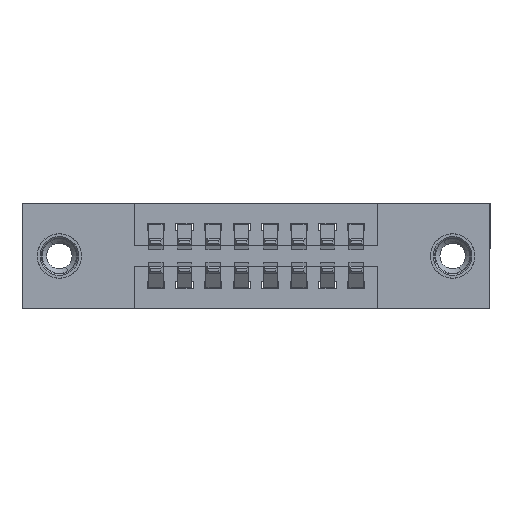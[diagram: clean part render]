
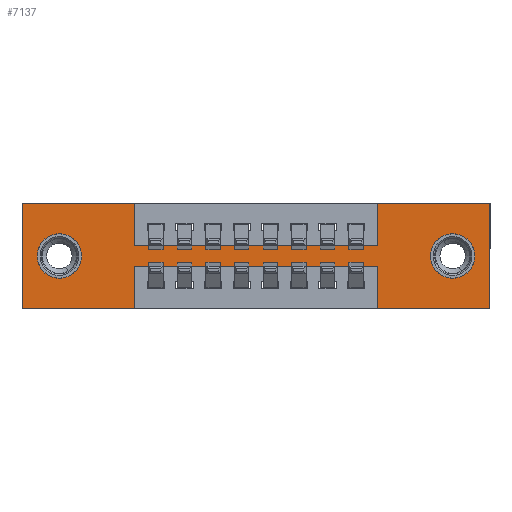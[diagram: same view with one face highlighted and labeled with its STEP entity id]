
A CAD part, front view. The second image highlights one B-rep face of the part: STEP entity #7137.
In plain terms, the highlighted planar face has unit normal (0, -1, 0).
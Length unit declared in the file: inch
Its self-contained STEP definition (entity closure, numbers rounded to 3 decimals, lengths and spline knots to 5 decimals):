
#36 = VECTOR ( 'NONE', #2842, 39.37008 ) ;
#48 = ORIENTED_EDGE ( 'NONE', *, *, #8321, .T. ) ;
#423 = CARTESIAN_POINT ( 'NONE',  ( 1.2425, 0., 0. ) ) ;
#436 = CARTESIAN_POINT ( 'NONE',  ( 0., 0., 0. ) ) ;
#591 = DIRECTION ( 'NONE',  ( 0., 0., 1. ) ) ;
#675 = VERTEX_POINT ( 'NONE', #4288 ) ;
#711 = CARTESIAN_POINT ( 'NONE',  ( 1.2425, 0., -0.22 ) ) ;
#812 = CARTESIAN_POINT ( 'NONE',  ( 0.3925, 0., -0.15 ) ) ;
#958 = CARTESIAN_POINT ( 'NONE',  ( 0.3925, 0., -0.37 ) ) ;
#1055 = EDGE_CURVE ( 'NONE', #2383, #12617, #11240, .T. ) ;
#1197 = VERTEX_POINT ( 'NONE', #436 ) ;
#1211 = DIRECTION ( 'NONE',  ( 0., 0., 1. ) ) ;
#1275 = CARTESIAN_POINT ( 'NONE',  ( 0.13, 0., -0.263 ) ) ;
#1289 = CARTESIAN_POINT ( 'NONE',  ( 0.3925, 0., -0.22 ) ) ;
#1409 = EDGE_CURVE ( 'NONE', #12295, #2345, #5709, .T. ) ;
#1460 = LINE ( 'NONE', #11836, #6264 ) ;
#1564 = DIRECTION ( 'NONE',  ( 1., 0., 0. ) ) ;
#1579 = ORIENTED_EDGE ( 'NONE', *, *, #4553, .F. ) ;
#1686 = ORIENTED_EDGE ( 'NONE', *, *, #5200, .F. ) ;
#1727 = DIRECTION ( 'NONE',  ( 0., 0., -1. ) ) ;
#1734 = FACE_BOUND ( 'NONE', #6515, .T. ) ;
#1882 = DIRECTION ( 'NONE',  ( 0., 0., -1. ) ) ;
#1994 = VECTOR ( 'NONE', #11374, 39.37008 ) ;
#1997 = CARTESIAN_POINT ( 'NONE',  ( 0., 0., -0.37 ) ) ;
#2053 = FACE_OUTER_BOUND ( 'NONE', #4636, .T. ) ;
#2105 = DIRECTION ( 'NONE',  ( -1., 0., 0. ) ) ;
#2143 = CARTESIAN_POINT ( 'NONE',  ( 1.2425, 0., 0. ) ) ;
#2266 = CARTESIAN_POINT ( 'NONE',  ( 0., 0., -0.37 ) ) ;
#2345 = VERTEX_POINT ( 'NONE', #8189 ) ;
#2347 = EDGE_CURVE ( 'NONE', #675, #11377, #6633, .T. ) ;
#2383 = VERTEX_POINT ( 'NONE', #6997 ) ;
#2524 = EDGE_CURVE ( 'NONE', #8164, #12295, #9024, .T. ) ;
#2536 = VECTOR ( 'NONE', #4565, 39.37008 ) ;
#2552 = DIRECTION ( 'NONE',  ( 0., 0., -1. ) ) ;
#2568 = CARTESIAN_POINT ( 'NONE',  ( 0., 0., 0. ) ) ;
#2617 = VECTOR ( 'NONE', #9044, 39.37008 ) ;
#2749 = DIRECTION ( 'NONE',  ( 0., 1., 0. ) ) ;
#2842 = DIRECTION ( 'NONE',  ( 0., 0., 1. ) ) ;
#2877 = AXIS2_PLACEMENT_3D ( 'NONE', #2935, #8913, #1882 ) ;
#2935 = CARTESIAN_POINT ( 'NONE',  ( 1.505, 0., -0.185 ) ) ;
#2956 = LINE ( 'NONE', #812, #2617 ) ;
#3151 = VERTEX_POINT ( 'NONE', #3806 ) ;
#3208 = VERTEX_POINT ( 'NONE', #2266 ) ;
#3241 = CIRCLE ( 'NONE', #2877, 0.078 ) ;
#3324 = CARTESIAN_POINT ( 'NONE',  ( 0.3925, 0., 0. ) ) ;
#3443 = ORIENTED_EDGE ( 'NONE', *, *, #10557, .T. ) ;
#3741 = EDGE_CURVE ( 'NONE', #6452, #8164, #2956, .T. ) ;
#3800 = DIRECTION ( 'NONE',  ( 1., 0., 0. ) ) ;
#3806 = CARTESIAN_POINT ( 'NONE',  ( 1.505, 0., -0.107 ) ) ;
#3946 = CIRCLE ( 'NONE', #6463, 0.078 ) ;
#4049 = EDGE_CURVE ( 'NONE', #2345, #675, #1460, .T. ) ;
#4132 = CARTESIAN_POINT ( 'NONE',  ( 0.3925, 0., -0.15 ) ) ;
#4146 = CARTESIAN_POINT ( 'NONE',  ( 0., 0., 0. ) ) ;
#4288 = CARTESIAN_POINT ( 'NONE',  ( 1.635, 0., -0.37 ) ) ;
#4373 = ORIENTED_EDGE ( 'NONE', *, *, #5862, .F. ) ;
#4392 = VERTEX_POINT ( 'NONE', #1275 ) ;
#4553 = EDGE_CURVE ( 'NONE', #11377, #7640, #10487, .T. ) ;
#4565 = DIRECTION ( 'NONE',  ( 0., 0., 1. ) ) ;
#4636 = EDGE_LOOP ( 'NONE', ( #6553, #10226, #1579, #6552, #11717, #11842, #8780, #10229, #5778, #13063, #4373, #1686 ) ) ;
#4665 = CARTESIAN_POINT ( 'NONE',  ( 0.3925, 0., 0. ) ) ;
#4873 = AXIS2_PLACEMENT_3D ( 'NONE', #7339, #5225, #11232 ) ;
#4968 = VERTEX_POINT ( 'NONE', #4665 ) ;
#4985 = CARTESIAN_POINT ( 'NONE',  ( 1.2425, 0., -0.15 ) ) ;
#5200 = EDGE_CURVE ( 'NONE', #12617, #3208, #5457, .T. ) ;
#5224 = CARTESIAN_POINT ( 'NONE',  ( 1.2425, 0., -0.37 ) ) ;
#5225 = DIRECTION ( 'NONE',  ( 0., -1., 0. ) ) ;
#5282 = CARTESIAN_POINT ( 'NONE',  ( 0., 0., -0.37 ) ) ;
#5457 = LINE ( 'NONE', #1997, #9731 ) ;
#5477 = CIRCLE ( 'NONE', #9786, 0.078 ) ;
#5508 = EDGE_CURVE ( 'NONE', #3151, #8769, #3241, .T. ) ;
#5697 = EDGE_LOOP ( 'NONE', ( #7759, #3443 ) ) ;
#5709 = LINE ( 'NONE', #2568, #8887 ) ;
#5765 = DIRECTION ( 'NONE',  ( 0., 1., 0. ) ) ;
#5778 = ORIENTED_EDGE ( 'NONE', *, *, #9629, .F. ) ;
#5862 = EDGE_CURVE ( 'NONE', #3208, #1197, #7328, .T. ) ;
#6264 = VECTOR ( 'NONE', #1727, 39.37008 ) ;
#6420 = CARTESIAN_POINT ( 'NONE',  ( 1.505, 0., -0.263 ) ) ;
#6452 = VERTEX_POINT ( 'NONE', #4132 ) ;
#6463 = AXIS2_PLACEMENT_3D ( 'NONE', #9794, #2749, #591 ) ;
#6515 = EDGE_LOOP ( 'NONE', ( #9899, #48 ) ) ;
#6552 = ORIENTED_EDGE ( 'NONE', *, *, #2347, .F. ) ;
#6553 = ORIENTED_EDGE ( 'NONE', *, *, #1055, .F. ) ;
#6633 = LINE ( 'NONE', #5282, #12322 ) ;
#6732 = CARTESIAN_POINT ( 'NONE',  ( 1.505, 0., -0.185 ) ) ;
#6997 = CARTESIAN_POINT ( 'NONE',  ( 0.3925, 0., -0.22 ) ) ;
#7137 = ADVANCED_FACE ( 'NONE', ( #1734, #9849, #2053 ), #7248, .T. ) ;
#7248 = PLANE ( 'NONE',  #4873 ) ;
#7328 = LINE ( 'NONE', #7796, #36 ) ;
#7335 = DIRECTION ( 'NONE',  ( 0., 1., 0. ) ) ;
#7339 = CARTESIAN_POINT ( 'NONE',  ( 0., 0., -0.37 ) ) ;
#7640 = VERTEX_POINT ( 'NONE', #711 ) ;
#7759 = ORIENTED_EDGE ( 'NONE', *, *, #9368, .T. ) ;
#7796 = CARTESIAN_POINT ( 'NONE',  ( 0., 0., 0. ) ) ;
#8077 = CIRCLE ( 'NONE', #12470, 0.078 ) ;
#8164 = VERTEX_POINT ( 'NONE', #4985 ) ;
#8189 = CARTESIAN_POINT ( 'NONE',  ( 1.635, 0., 0. ) ) ;
#8197 = LINE ( 'NONE', #1289, #11671 ) ;
#8321 = EDGE_CURVE ( 'NONE', #8769, #3151, #8077, .T. ) ;
#8427 = DIRECTION ( 'NONE',  ( -1., 0., 0. ) ) ;
#8769 = VERTEX_POINT ( 'NONE', #6420 ) ;
#8780 = ORIENTED_EDGE ( 'NONE', *, *, #2524, .F. ) ;
#8887 = VECTOR ( 'NONE', #1564, 39.37008 ) ;
#8913 = DIRECTION ( 'NONE',  ( 0., 1., 0. ) ) ;
#9024 = LINE ( 'NONE', #2143, #9646 ) ;
#9044 = DIRECTION ( 'NONE',  ( 1., 0., 0. ) ) ;
#9144 = EDGE_CURVE ( 'NONE', #7640, #2383, #8197, .T. ) ;
#9368 = EDGE_CURVE ( 'NONE', #10683, #4392, #3946, .T. ) ;
#9629 = EDGE_CURVE ( 'NONE', #4968, #6452, #10265, .T. ) ;
#9646 = VECTOR ( 'NONE', #12380, 39.37008 ) ;
#9662 = DIRECTION ( 'NONE',  ( 0., 0., -1. ) ) ;
#9731 = VECTOR ( 'NONE', #11190, 39.37008 ) ;
#9786 = AXIS2_PLACEMENT_3D ( 'NONE', #11480, #7335, #1211 ) ;
#9794 = CARTESIAN_POINT ( 'NONE',  ( 0.13, 0., -0.185 ) ) ;
#9849 = FACE_BOUND ( 'NONE', #5697, .T. ) ;
#9899 = ORIENTED_EDGE ( 'NONE', *, *, #5508, .T. ) ;
#10226 = ORIENTED_EDGE ( 'NONE', *, *, #9144, .F. ) ;
#10229 = ORIENTED_EDGE ( 'NONE', *, *, #3741, .F. ) ;
#10265 = LINE ( 'NONE', #3324, #1994 ) ;
#10487 = LINE ( 'NONE', #5224, #2536 ) ;
#10557 = EDGE_CURVE ( 'NONE', #4392, #10683, #5477, .T. ) ;
#10683 = VERTEX_POINT ( 'NONE', #11868 ) ;
#10781 = VECTOR ( 'NONE', #2552, 39.37008 ) ;
#11190 = DIRECTION ( 'NONE',  ( -1., 0., 0. ) ) ;
#11232 = DIRECTION ( 'NONE',  ( 0., 0., -1. ) ) ;
#11240 = LINE ( 'NONE', #11588, #10781 ) ;
#11374 = DIRECTION ( 'NONE',  ( 0., 0., -1. ) ) ;
#11377 = VERTEX_POINT ( 'NONE', #12389 ) ;
#11480 = CARTESIAN_POINT ( 'NONE',  ( 0.13, 0., -0.185 ) ) ;
#11588 = CARTESIAN_POINT ( 'NONE',  ( 0.3925, 0., -0.37 ) ) ;
#11671 = VECTOR ( 'NONE', #8427, 39.37008 ) ;
#11717 = ORIENTED_EDGE ( 'NONE', *, *, #4049, .F. ) ;
#11836 = CARTESIAN_POINT ( 'NONE',  ( 1.635, 0., 0. ) ) ;
#11842 = ORIENTED_EDGE ( 'NONE', *, *, #1409, .F. ) ;
#11845 = LINE ( 'NONE', #4146, #13115 ) ;
#11868 = CARTESIAN_POINT ( 'NONE',  ( 0.13, 0., -0.107 ) ) ;
#12295 = VERTEX_POINT ( 'NONE', #423 ) ;
#12322 = VECTOR ( 'NONE', #2105, 39.37008 ) ;
#12380 = DIRECTION ( 'NONE',  ( 0., 0., 1. ) ) ;
#12389 = CARTESIAN_POINT ( 'NONE',  ( 1.2425, 0., -0.37 ) ) ;
#12408 = EDGE_CURVE ( 'NONE', #1197, #4968, #11845, .T. ) ;
#12470 = AXIS2_PLACEMENT_3D ( 'NONE', #6732, #5765, #9662 ) ;
#12617 = VERTEX_POINT ( 'NONE', #958 ) ;
#13063 = ORIENTED_EDGE ( 'NONE', *, *, #12408, .F. ) ;
#13115 = VECTOR ( 'NONE', #3800, 39.37008 ) ;
